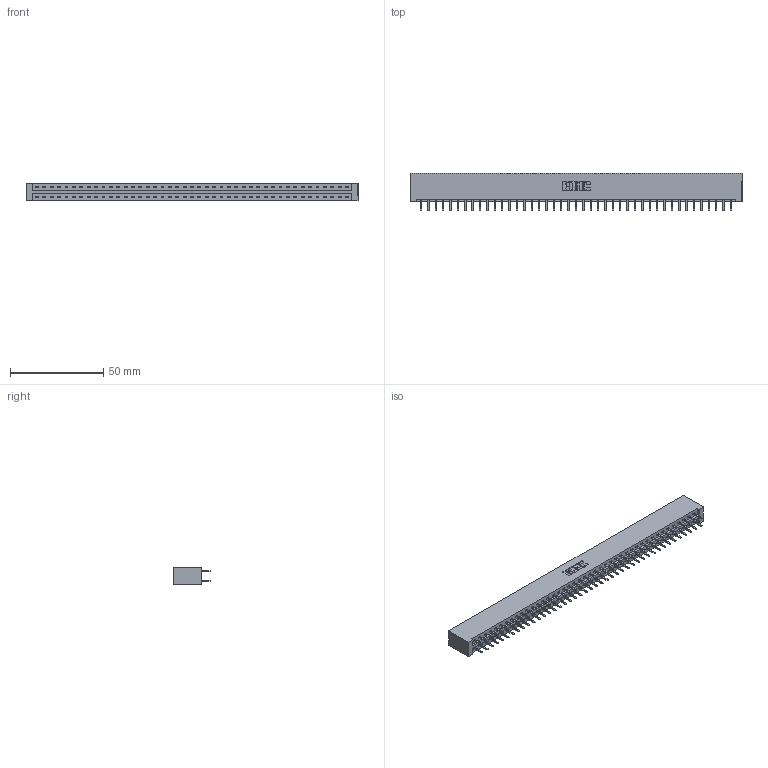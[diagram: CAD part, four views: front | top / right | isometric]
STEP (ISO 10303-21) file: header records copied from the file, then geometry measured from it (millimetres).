
FILE_DESCRIPTION (( 'STEP AP203' ), '1' );
FILE_NAME ('387-086-520-201.STEP', '2019-10-23T02:41:40', ( '' ), ( '' ), 'SwSTEP 2.0', 'SolidWorks 2016', '' );
FILE_SCHEMA (( 'CONFIG_CONTROL_DESIGN' ));
Length unit declared in the file: inch
Products named in the file (3): 345-292-001_345-293-120; 387-086-520-201; 337 Part_No Mounting Lugs
Assembly tree (87 placements, depth 2):
  387-086-520-201
    337 Part_No Mounting Lugs
    345-292-001_345-293-120  x86
Bounding box: 178.26 x 20.02 x 9.4 mm (x, y, z)
Volume: 19522.4 mm3; surface area: 22028.1 mm2
Topology: 87 solids, 87 shells, 5094 faces, 14821 edges, 9650 vertices
Faces by surface type: plane 3506, cylinder 1588
Entity records: 33047 total; most frequent: CARTESIAN_POINT 5578, ORIENTED_EDGE 5502, DIRECTION 4723, EDGE_CURVE 2751, VECTOR 2627, LINE 2627, VERTEX_POINT 1830, AXIS2_PLACEMENT_3D 1048
